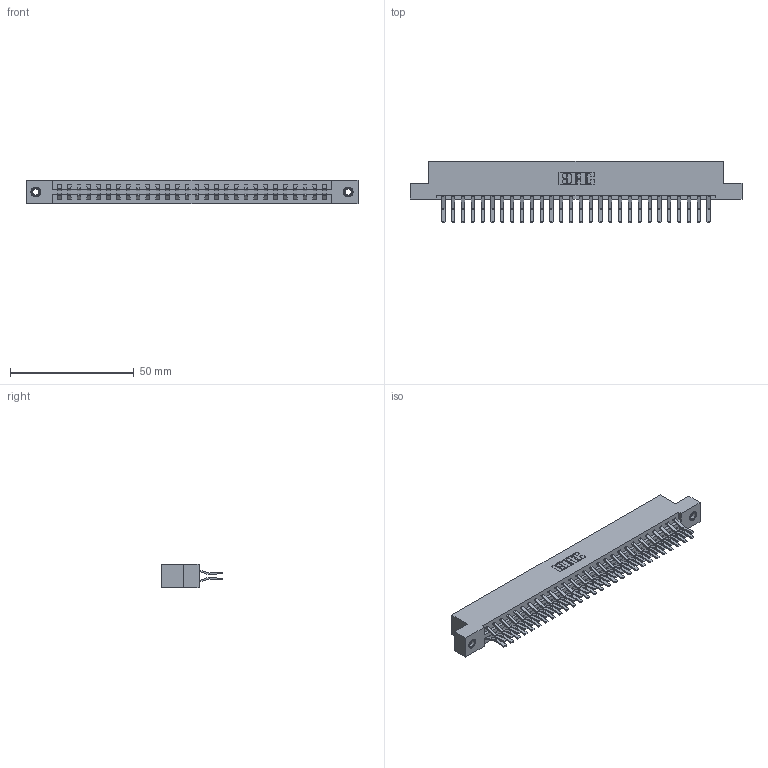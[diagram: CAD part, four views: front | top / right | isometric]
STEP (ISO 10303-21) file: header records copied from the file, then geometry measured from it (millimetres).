
FILE_DESCRIPTION (( 'STEP AP203' ), '1' );
FILE_NAME ('387-056-560-207.STEP', '2019-10-19T08:07:53', ( '' ), ( '' ), 'SwSTEP 2.0', 'SolidWorks 2016', '' );
FILE_SCHEMA (( 'CONFIG_CONTROL_DESIGN' ));
Length unit declared in the file: inch
Products named in the file (4): 337 Part_Flush Mounting Lugs - 0.156 Dia-TI; 345-292-001_560 Tail; 345-250-001_345-250-005-103; 387-056-560-207
Assembly tree (59 placements, depth 2):
  387-056-560-207
    337 Part_Flush Mounting Lugs - 0.156 Dia-TI
    345-292-001_560 Tail  x56
    345-250-001_345-250-005-103  x2
Bounding box: 133.96 x 24.78 x 9.4 mm (x, y, z)
Volume: 14284.9 mm3; surface area: 17111.4 mm2
Topology: 59 solids, 59 shells, 3310 faces, 9799 edges, 6450 vertices
Faces by surface type: plane 2230, cylinder 1064, cone 12, torus 4
Entity records: 24794 total; most frequent: CARTESIAN_POINT 4169, ORIENTED_EDGE 4098, DIRECTION 3607, EDGE_CURVE 2049, LINE 1897, VECTOR 1897, VERTEX_POINT 1360, AXIS2_PLACEMENT_3D 855
